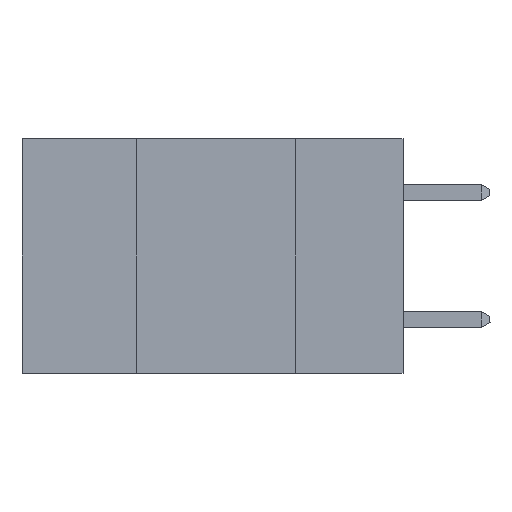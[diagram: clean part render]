
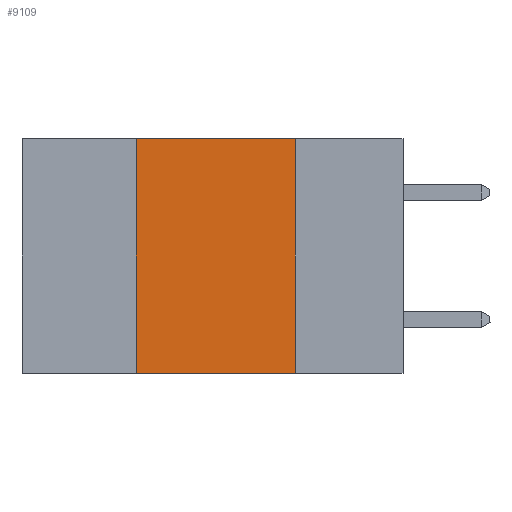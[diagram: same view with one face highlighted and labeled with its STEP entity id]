
A CAD part, left-side view. The second image highlights one B-rep face of the part: STEP entity #9109.
In plain terms, the highlighted planar face has unit normal (-1, 0, 0).
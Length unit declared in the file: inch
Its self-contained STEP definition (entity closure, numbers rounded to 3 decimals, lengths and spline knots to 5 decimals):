
#818 = LINE ( 'NONE', #24204, #28647 ) ;
#1667 = ORIENTED_EDGE ( 'NONE', *, *, #10098, .F. ) ;
#2712 = DIRECTION ( 'NONE',  ( 0., 0., -1. ) ) ;
#2878 = EDGE_CURVE ( 'NONE', #34561, #8204, #22493, .T. ) ;
#3223 = ORIENTED_EDGE ( 'NONE', *, *, #36724, .F. ) ;
#4338 = CARTESIAN_POINT ( 'NONE',  ( 0., 0.6, -0.37 ) ) ;
#5370 = VECTOR ( 'NONE', #22989, 39.37008 ) ;
#5816 = CARTESIAN_POINT ( 'NONE',  ( 0., 0.42, 0. ) ) ;
#5938 = AXIS2_PLACEMENT_3D ( 'NONE', #18242, #17848, #2712 ) ;
#7462 = CARTESIAN_POINT ( 'NONE',  ( 0., 0.42, 0. ) ) ;
#8204 = VERTEX_POINT ( 'NONE', #22100 ) ;
#8302 = FACE_OUTER_BOUND ( 'NONE', #14040, .T. ) ;
#9109 = ADVANCED_FACE ( 'NONE', ( #8302 ), #36544, .F. ) ;
#9375 = ORIENTED_EDGE ( 'NONE', *, *, #14061, .F. ) ;
#10098 = EDGE_CURVE ( 'NONE', #34561, #19063, #38720, .T. ) ;
#11083 = VECTOR ( 'NONE', #25407, 39.37008 ) ;
#12014 = VECTOR ( 'NONE', #22753, 39.37008 ) ;
#12897 = CARTESIAN_POINT ( 'NONE',  ( 0., 0.17, 0. ) ) ;
#14040 = EDGE_LOOP ( 'NONE', ( #3223, #9375, #1667, #21585 ) ) ;
#14061 = EDGE_CURVE ( 'NONE', #19063, #16560, #818, .T. ) ;
#15794 = DIRECTION ( 'NONE',  ( 0., -1., 0. ) ) ;
#16560 = VERTEX_POINT ( 'NONE', #34335 ) ;
#17848 = DIRECTION ( 'NONE',  ( 1., 0., 0. ) ) ;
#18242 = CARTESIAN_POINT ( 'NONE',  ( 0., 0.6, 0. ) ) ;
#19063 = VERTEX_POINT ( 'NONE', #5816 ) ;
#20116 = LINE ( 'NONE', #12897, #11083 ) ;
#21585 = ORIENTED_EDGE ( 'NONE', *, *, #2878, .T. ) ;
#22100 = CARTESIAN_POINT ( 'NONE',  ( 0., 0.17, -0.37 ) ) ;
#22493 = LINE ( 'NONE', #4338, #5370 ) ;
#22753 = DIRECTION ( 'NONE',  ( 0., 0., 1. ) ) ;
#22989 = DIRECTION ( 'NONE',  ( 0., -1., 0. ) ) ;
#24204 = CARTESIAN_POINT ( 'NONE',  ( 0., 0.6, 0. ) ) ;
#24349 = CARTESIAN_POINT ( 'NONE',  ( 0., 0.42, -0.37 ) ) ;
#25407 = DIRECTION ( 'NONE',  ( 0., 0., -1. ) ) ;
#28647 = VECTOR ( 'NONE', #15794, 39.37008 ) ;
#34335 = CARTESIAN_POINT ( 'NONE',  ( 0., 0.17, 0. ) ) ;
#34561 = VERTEX_POINT ( 'NONE', #24349 ) ;
#36544 = PLANE ( 'NONE',  #5938 ) ;
#36724 = EDGE_CURVE ( 'NONE', #16560, #8204, #20116, .T. ) ;
#38720 = LINE ( 'NONE', #7462, #12014 ) ;
